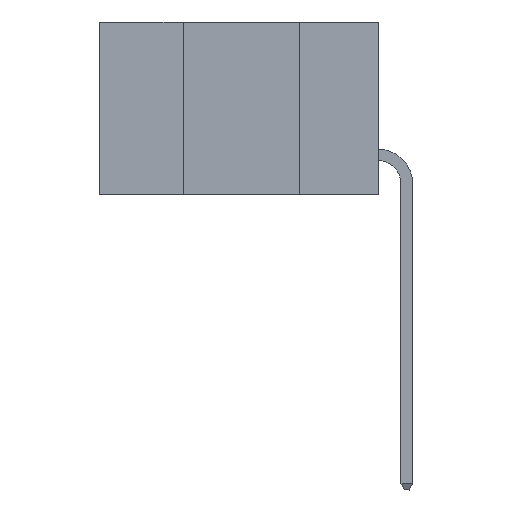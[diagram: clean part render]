
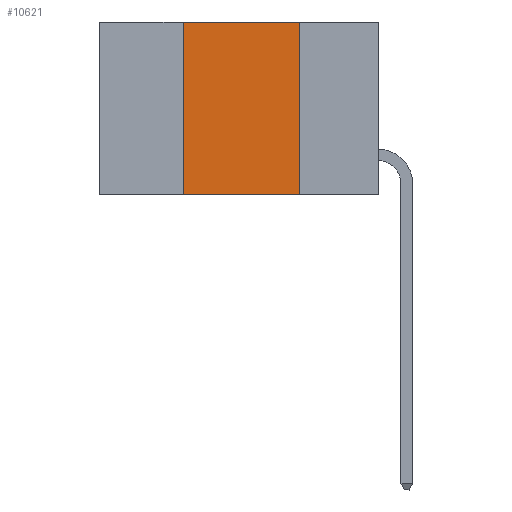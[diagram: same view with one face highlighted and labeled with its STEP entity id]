
A CAD part, left-side view. The second image highlights one B-rep face of the part: STEP entity #10621.
In plain terms, the highlighted planar face has unit normal (-1, 0, 0).
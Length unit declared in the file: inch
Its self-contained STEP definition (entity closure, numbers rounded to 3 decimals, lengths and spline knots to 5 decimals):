
#959 = CARTESIAN_POINT ( 'NONE',  ( 0., 0.6, -0.37 ) ) ;
#1958 = AXIS2_PLACEMENT_3D ( 'NONE', #2631, #25682, #21207 ) ;
#2631 = CARTESIAN_POINT ( 'NONE',  ( 0., 0.6, 0. ) ) ;
#3432 = EDGE_CURVE ( 'NONE', #10228, #25873, #19180, .T. ) ;
#4152 = VECTOR ( 'NONE', #15606, 39.37008 ) ;
#6294 = VECTOR ( 'NONE', #13134, 39.37008 ) ;
#6517 = CARTESIAN_POINT ( 'NONE',  ( 0., 0.17, 0. ) ) ;
#6670 = PLANE ( 'NONE',  #1958 ) ;
#7324 = CARTESIAN_POINT ( 'NONE',  ( 0., 0.42, -0.37 ) ) ;
#7697 = ORIENTED_EDGE ( 'NONE', *, *, #8408, .F. ) ;
#8364 = CARTESIAN_POINT ( 'NONE',  ( 0., 0.17, 0. ) ) ;
#8408 = EDGE_CURVE ( 'NONE', #10228, #22096, #11342, .T. ) ;
#10185 = LINE ( 'NONE', #11027, #6294 ) ;
#10213 = ORIENTED_EDGE ( 'NONE', *, *, #22991, .F. ) ;
#10228 = VERTEX_POINT ( 'NONE', #7324 ) ;
#10621 = ADVANCED_FACE ( 'NONE', ( #14958 ), #6670, .F. ) ;
#11027 = CARTESIAN_POINT ( 'NONE',  ( 0., 0.6, 0. ) ) ;
#11032 = ORIENTED_EDGE ( 'NONE', *, *, #24158, .F. ) ;
#11342 = LINE ( 'NONE', #15717, #16290 ) ;
#12420 = VECTOR ( 'NONE', #19315, 39.37008 ) ;
#13134 = DIRECTION ( 'NONE',  ( 0., -1., 0. ) ) ;
#14958 = FACE_OUTER_BOUND ( 'NONE', #16802, .T. ) ;
#15606 = DIRECTION ( 'NONE',  ( 0., -1., 0. ) ) ;
#15717 = CARTESIAN_POINT ( 'NONE',  ( 0., 0.42, 0. ) ) ;
#16290 = VECTOR ( 'NONE', #24012, 39.37008 ) ;
#16400 = CARTESIAN_POINT ( 'NONE',  ( 0., 0.42, 0. ) ) ;
#16802 = EDGE_LOOP ( 'NONE', ( #11032, #10213, #7697, #17300 ) ) ;
#17026 = VERTEX_POINT ( 'NONE', #8364 ) ;
#17300 = ORIENTED_EDGE ( 'NONE', *, *, #3432, .T. ) ;
#19180 = LINE ( 'NONE', #959, #4152 ) ;
#19315 = DIRECTION ( 'NONE',  ( 0., 0., -1. ) ) ;
#21207 = DIRECTION ( 'NONE',  ( 0., 0., -1. ) ) ;
#21610 = CARTESIAN_POINT ( 'NONE',  ( 0., 0.17, -0.37 ) ) ;
#22096 = VERTEX_POINT ( 'NONE', #16400 ) ;
#22991 = EDGE_CURVE ( 'NONE', #22096, #17026, #10185, .T. ) ;
#24012 = DIRECTION ( 'NONE',  ( 0., 0., 1. ) ) ;
#24158 = EDGE_CURVE ( 'NONE', #17026, #25873, #26845, .T. ) ;
#25682 = DIRECTION ( 'NONE',  ( 1., 0., 0. ) ) ;
#25873 = VERTEX_POINT ( 'NONE', #21610 ) ;
#26845 = LINE ( 'NONE', #6517, #12420 ) ;
